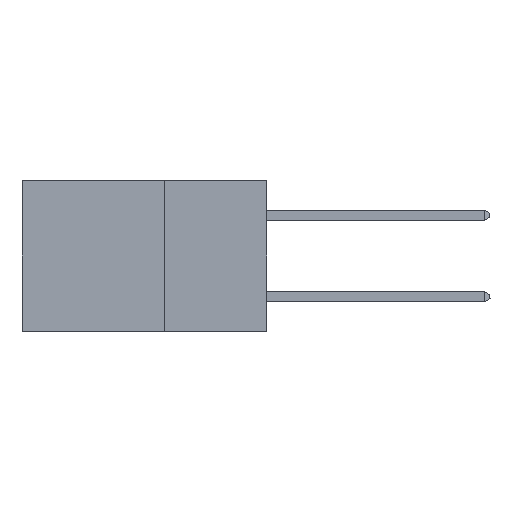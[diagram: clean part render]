
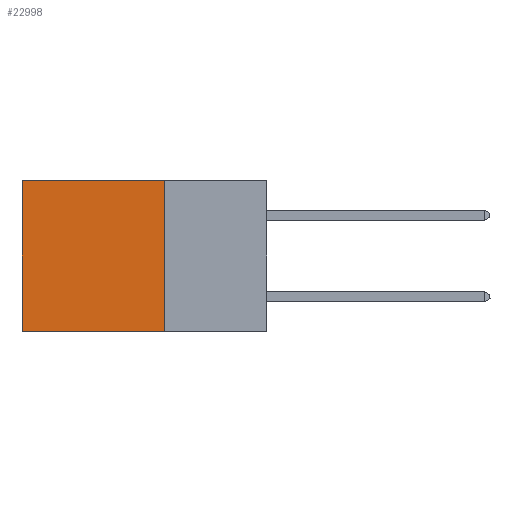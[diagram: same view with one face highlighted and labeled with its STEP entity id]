
A CAD part, left-side view. The second image highlights one B-rep face of the part: STEP entity #22998.
In plain terms, the highlighted planar face has unit normal (-1, 0, 0).
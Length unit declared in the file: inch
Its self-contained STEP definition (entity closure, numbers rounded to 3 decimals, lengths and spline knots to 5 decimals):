
#68 = CARTESIAN_POINT ( 'NONE',  ( 0.2875, 0.25, 0. ) ) ;
#2890 = CARTESIAN_POINT ( 'NONE',  ( 0.2875, 0.25, -0.37 ) ) ;
#3097 = VERTEX_POINT ( 'NONE', #12453 ) ;
#3852 = DIRECTION ( 'NONE',  ( 1., 0., 0. ) ) ;
#4842 = CARTESIAN_POINT ( 'NONE',  ( 0.2875, 0.25, 0. ) ) ;
#6894 = VERTEX_POINT ( 'NONE', #9460 ) ;
#7503 = VECTOR ( 'NONE', #18910, 39.37008 ) ;
#7886 = DIRECTION ( 'NONE',  ( 0., 0., -1. ) ) ;
#8445 = VECTOR ( 'NONE', #14013, 39.37008 ) ;
#8902 = LINE ( 'NONE', #4842, #11468 ) ;
#9460 = CARTESIAN_POINT ( 'NONE',  ( 0.2875, 0.6, 0. ) ) ;
#9917 = CARTESIAN_POINT ( 'NONE',  ( 0.2875, 0.25, 0. ) ) ;
#10171 = ORIENTED_EDGE ( 'NONE', *, *, #23151, .T. ) ;
#10303 = ORIENTED_EDGE ( 'NONE', *, *, #18091, .T. ) ;
#10372 = ORIENTED_EDGE ( 'NONE', *, *, #10841, .F. ) ;
#10841 = EDGE_CURVE ( 'NONE', #22375, #10881, #8902, .T. ) ;
#10881 = VERTEX_POINT ( 'NONE', #2890 ) ;
#10888 = ORIENTED_EDGE ( 'NONE', *, *, #25145, .F. ) ;
#11468 = VECTOR ( 'NONE', #23507, 39.37008 ) ;
#12453 = CARTESIAN_POINT ( 'NONE',  ( 0.2875, 0.6, -0.37 ) ) ;
#12904 = LINE ( 'NONE', #20970, #7503 ) ;
#13359 = EDGE_LOOP ( 'NONE', ( #10171, #10888, #10372, #10303 ) ) ;
#13550 = LINE ( 'NONE', #14828, #21296 ) ;
#13574 = LINE ( 'NONE', #9917, #8445 ) ;
#14013 = DIRECTION ( 'NONE',  ( 0., 1., 0. ) ) ;
#14362 = AXIS2_PLACEMENT_3D ( 'NONE', #16210, #3852, #7886 ) ;
#14828 = CARTESIAN_POINT ( 'NONE',  ( 0.2875, 0.25, -0.37 ) ) ;
#16210 = CARTESIAN_POINT ( 'NONE',  ( 0.2875, 0.25, 0. ) ) ;
#18091 = EDGE_CURVE ( 'NONE', #22375, #6894, #13574, .T. ) ;
#18910 = DIRECTION ( 'NONE',  ( 0., 0., -1. ) ) ;
#20187 = PLANE ( 'NONE',  #14362 ) ;
#20334 = FACE_OUTER_BOUND ( 'NONE', #13359, .T. ) ;
#20970 = CARTESIAN_POINT ( 'NONE',  ( 0.2875, 0.6, 0. ) ) ;
#21296 = VECTOR ( 'NONE', #23125, 39.37008 ) ;
#22375 = VERTEX_POINT ( 'NONE', #68 ) ;
#22998 = ADVANCED_FACE ( 'NONE', ( #20334 ), #20187, .F. ) ;
#23125 = DIRECTION ( 'NONE',  ( 0., 1., 0. ) ) ;
#23151 = EDGE_CURVE ( 'NONE', #6894, #3097, #12904, .T. ) ;
#23507 = DIRECTION ( 'NONE',  ( 0., 0., -1. ) ) ;
#25145 = EDGE_CURVE ( 'NONE', #10881, #3097, #13550, .T. ) ;
